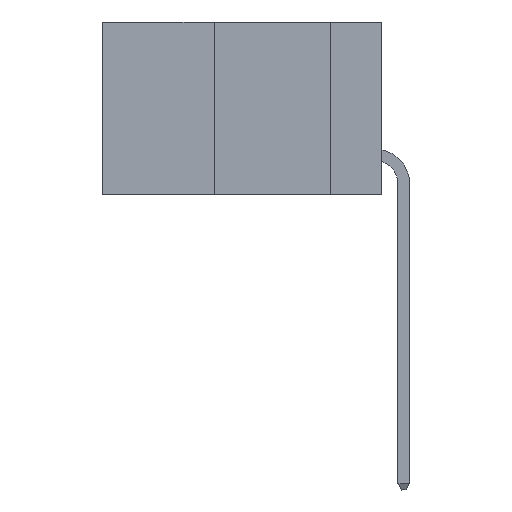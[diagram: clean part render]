
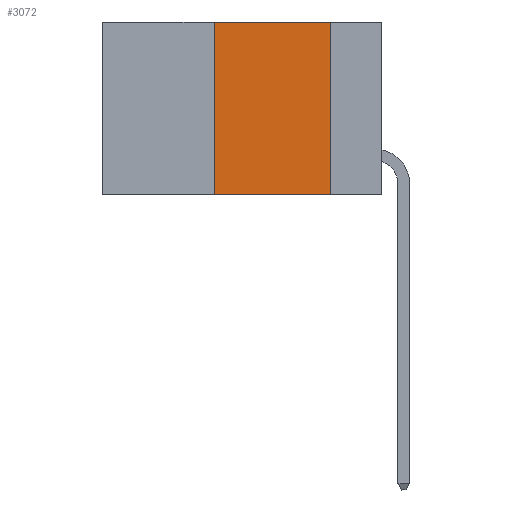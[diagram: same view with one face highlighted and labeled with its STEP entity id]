
A CAD part, left-side view. The second image highlights one B-rep face of the part: STEP entity #3072.
In plain terms, the highlighted planar face has unit normal (-1, 0, 0).
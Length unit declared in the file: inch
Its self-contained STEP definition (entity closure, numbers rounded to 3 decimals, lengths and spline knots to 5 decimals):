
#377 = VERTEX_POINT ( 'NONE', #5516 ) ;
#988 = EDGE_CURVE ( 'NONE', #16010, #3846, #8873, .T. ) ;
#1653 = LINE ( 'NONE', #11587, #12632 ) ;
#3072 = ADVANCED_FACE ( 'NONE', ( #17974 ), #10292, .F. ) ;
#3846 = VERTEX_POINT ( 'NONE', #11474 ) ;
#4537 = ORIENTED_EDGE ( 'NONE', *, *, #988, .T. ) ;
#4626 = EDGE_CURVE ( 'NONE', #15300, #377, #13052, .T. ) ;
#5124 = ORIENTED_EDGE ( 'NONE', *, *, #13599, .F. ) ;
#5516 = CARTESIAN_POINT ( 'NONE',  ( 0., 0.11, 0. ) ) ;
#6864 = VECTOR ( 'NONE', #8665, 39.37008 ) ;
#7533 = DIRECTION ( 'NONE',  ( 1., 0., 0. ) ) ;
#8566 = DIRECTION ( 'NONE',  ( 0., -1., 0. ) ) ;
#8665 = DIRECTION ( 'NONE',  ( 0., -1., 0. ) ) ;
#8873 = LINE ( 'NONE', #30927, #30104 ) ;
#10124 = EDGE_LOOP ( 'NONE', ( #5124, #27544, #18882, #4537 ) ) ;
#10292 = PLANE ( 'NONE',  #10654 ) ;
#10615 = CARTESIAN_POINT ( 'NONE',  ( 0., 0.6, 0. ) ) ;
#10654 = AXIS2_PLACEMENT_3D ( 'NONE', #29892, #7533, #17508 ) ;
#10742 = EDGE_CURVE ( 'NONE', #16010, #15300, #1653, .T. ) ;
#11474 = CARTESIAN_POINT ( 'NONE',  ( 0., 0.11, -0.37 ) ) ;
#11587 = CARTESIAN_POINT ( 'NONE',  ( 0., 0.36, 0. ) ) ;
#12632 = VECTOR ( 'NONE', #21564, 39.37008 ) ;
#13052 = LINE ( 'NONE', #10615, #6864 ) ;
#13599 = EDGE_CURVE ( 'NONE', #377, #3846, #16115, .T. ) ;
#13768 = VECTOR ( 'NONE', #16447, 39.37008 ) ;
#13941 = CARTESIAN_POINT ( 'NONE',  ( 0., 0.36, 0. ) ) ;
#15300 = VERTEX_POINT ( 'NONE', #13941 ) ;
#16010 = VERTEX_POINT ( 'NONE', #22009 ) ;
#16115 = LINE ( 'NONE', #23914, #13768 ) ;
#16447 = DIRECTION ( 'NONE',  ( 0., 0., -1. ) ) ;
#17508 = DIRECTION ( 'NONE',  ( 0., 0., -1. ) ) ;
#17974 = FACE_OUTER_BOUND ( 'NONE', #10124, .T. ) ;
#18882 = ORIENTED_EDGE ( 'NONE', *, *, #10742, .F. ) ;
#21564 = DIRECTION ( 'NONE',  ( 0., 0., 1. ) ) ;
#22009 = CARTESIAN_POINT ( 'NONE',  ( 0., 0.36, -0.37 ) ) ;
#23914 = CARTESIAN_POINT ( 'NONE',  ( 0., 0.11, 0. ) ) ;
#27544 = ORIENTED_EDGE ( 'NONE', *, *, #4626, .F. ) ;
#29892 = CARTESIAN_POINT ( 'NONE',  ( 0., 0.6, 0. ) ) ;
#30104 = VECTOR ( 'NONE', #8566, 39.37008 ) ;
#30927 = CARTESIAN_POINT ( 'NONE',  ( 0., 0.6, -0.37 ) ) ;
